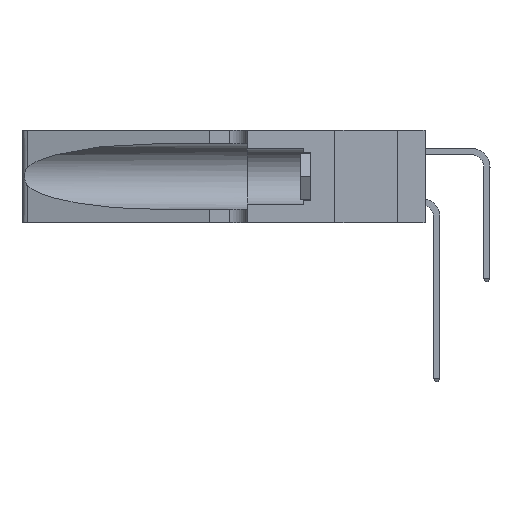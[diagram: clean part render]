
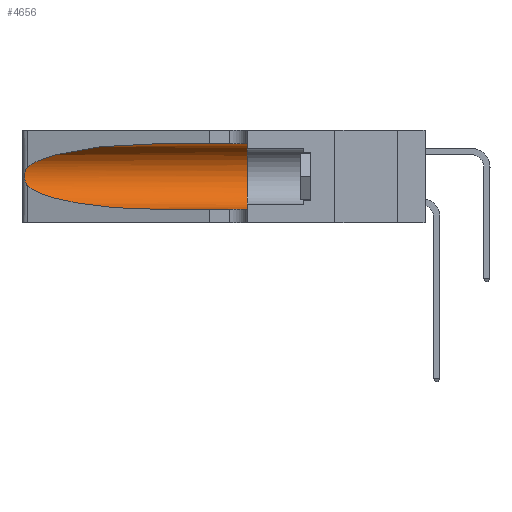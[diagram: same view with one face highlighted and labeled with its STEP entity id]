
A CAD part, left-side view. The second image highlights one B-rep face of the part: STEP entity #4656.
In plain terms, the highlighted cylindrical face has radius 3.308 mm (diameter 6.617 mm), a partial arc.
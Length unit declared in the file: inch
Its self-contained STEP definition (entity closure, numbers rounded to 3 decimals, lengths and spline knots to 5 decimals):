
#971 = EDGE_CURVE ( 'NONE', #30730, #7236, #8012, .T. ) ;
#1687 = VERTEX_POINT ( 'NONE', #6755 ) ;
#1723 = CARTESIAN_POINT ( 'NONE',  ( 0.1305, 1.61858, 0.05475 ) ) ;
#2503 = VECTOR ( 'NONE', #32444, 39.37008 ) ;
#2796 = VERTEX_POINT ( 'NONE', #14211 ) ;
#4023 = CARTESIAN_POINT ( 'NONE',  ( 0.1305, 0.72297, 0.31525 ) ) ;
#4656 = ADVANCED_FACE ( 'NONE', ( #18429 ), #18803, .F. ) ;
#6582 = EDGE_CURVE ( 'NONE', #15740, #2796, #26088, .T. ) ;
#6755 = CARTESIAN_POINT ( 'NONE',  ( 0.1305, 0.35, 0.31525 ) ) ;
#7236 = VERTEX_POINT ( 'NONE', #12376 ) ;
#7680 = CARTESIAN_POINT ( 'NONE',  ( 0.25487, 1.22718, 0.14631 ) ) ;
#8012 =( BOUNDED_CURVE ( )  B_SPLINE_CURVE ( 3, ( #4023, #9472, #24943, #17368 ),
 .UNSPECIFIED., .F., .T. ) 
 B_SPLINE_CURVE_WITH_KNOTS ( ( 4, 4 ),
 ( 1.5708, 2.84003 ),
 .UNSPECIFIED. ) 
 CURVE ( )  GEOMETRIC_REPRESENTATION_ITEM ( )  RATIONAL_B_SPLINE_CURVE ( ( 1., 0.87, 0.87, 1. ) ) 
 REPRESENTATION_ITEM ( '' )  );
#9037 = CIRCLE ( 'NONE', #13797, 0.13025 ) ;
#9049 = DIRECTION ( 'NONE',  ( 0., 0., 1. ) ) ;
#9266 = CARTESIAN_POINT ( 'NONE',  ( 0.1305, 0.72297, 0.31525 ) ) ;
#9472 = CARTESIAN_POINT ( 'NONE',  ( 0.18966, 0.96281, 0.31525 ) ) ;
#10345 = ORIENTED_EDGE ( 'NONE', *, *, #21087, .T. ) ;
#11598 = LINE ( 'NONE', #26749, #31952 ) ;
#11802 = CARTESIAN_POINT ( 'NONE',  ( 0.26075, 1.23896, 0.19203 ) ) ;
#11924 = CARTESIAN_POINT ( 'NONE',  ( 0.25639, 1.23186, 0.15144 ) ) ;
#12041 = CARTESIAN_POINT ( 'NONE',  ( 0.25487, 1.22718, 0.22369 ) ) ;
#12376 = CARTESIAN_POINT ( 'NONE',  ( 0.25487, 1.22718, 0.22369 ) ) ;
#12915 = EDGE_CURVE ( 'NONE', #30730, #1687, #11598, .T. ) ;
#13797 = AXIS2_PLACEMENT_3D ( 'NONE', #30279, #24888, #9049 ) ;
#13866 = CARTESIAN_POINT ( 'NONE',  ( 0.25487, 1.22718, 0.14631 ) ) ;
#13899 = DIRECTION ( 'NONE',  ( 0., -1., 0. ) ) ;
#14119 = CARTESIAN_POINT ( 'NONE',  ( 0.1305, 1.61858, 0.185 ) ) ;
#14211 = CARTESIAN_POINT ( 'NONE',  ( 0.1305, 0.35, 0.05475 ) ) ;
#15256 =( BOUNDED_CURVE ( )  B_SPLINE_CURVE ( 3, ( #7680, #18378, #34017, #26201 ),
 .UNSPECIFIED., .F., .F. ) 
 B_SPLINE_CURVE_WITH_KNOTS ( ( 4, 4 ),
 ( 3.44316, 4.71239 ),
 .UNSPECIFIED. ) 
 CURVE ( )  GEOMETRIC_REPRESENTATION_ITEM ( )  RATIONAL_B_SPLINE_CURVE ( ( 1., 0.87, 0.87, 1. ) ) 
 REPRESENTATION_ITEM ( '' )  );
#15740 = VERTEX_POINT ( 'NONE', #21078 ) ;
#16874 = EDGE_CURVE ( 'NONE', #7236, #31342, #18451, .T. ) ;
#16885 = ORIENTED_EDGE ( 'NONE', *, *, #12915, .F. ) ;
#17141 = CARTESIAN_POINT ( 'NONE',  ( 0.25789, 1.23486, 0.15765 ) ) ;
#17258 = CARTESIAN_POINT ( 'NONE',  ( 0.26017, 1.23833, 0.17102 ) ) ;
#17368 = CARTESIAN_POINT ( 'NONE',  ( 0.25487, 1.22718, 0.22369 ) ) ;
#18378 = CARTESIAN_POINT ( 'NONE',  ( 0.2373, 1.15595, 0.08982 ) ) ;
#18429 = FACE_OUTER_BOUND ( 'NONE', #32497, .T. ) ;
#18451 = B_SPLINE_CURVE_WITH_KNOTS ( 'NONE', 3,
 ( #12041, #24957, #27506, #27621, #22561, #25093, #11802, #30221, #17258, #30351, #17141, #11924, #27741, #30464 ),
 .UNSPECIFIED., .F., .F.,
 ( 4, 2, 2, 2, 2, 2, 4 ),
 ( 0., 0.00027, 0.00053, 0.00107, 0.0016, 0.00187, 0.00214 ),
 .UNSPECIFIED. ) ;
#18803 = CYLINDRICAL_SURFACE ( 'NONE', #33532, 0.13025 ) ;
#20384 = EDGE_CURVE ( 'NONE', #1687, #2796, #9037, .T. ) ;
#21078 = CARTESIAN_POINT ( 'NONE',  ( 0.1305, 0.72297, 0.05475 ) ) ;
#21087 = EDGE_CURVE ( 'NONE', #31342, #15740, #15256, .T. ) ;
#21212 = ORIENTED_EDGE ( 'NONE', *, *, #6582, .T. ) ;
#22356 = DIRECTION ( 'NONE',  ( 0., -1., 0. ) ) ;
#22364 = ORIENTED_EDGE ( 'NONE', *, *, #16874, .T. ) ;
#22561 = CARTESIAN_POINT ( 'NONE',  ( 0.25854, 1.2359, 0.20912 ) ) ;
#24888 = DIRECTION ( 'NONE',  ( 0., 1., 0. ) ) ;
#24943 = CARTESIAN_POINT ( 'NONE',  ( 0.2373, 1.15595, 0.28018 ) ) ;
#24957 = CARTESIAN_POINT ( 'NONE',  ( 0.25555, 1.22994, 0.2215 ) ) ;
#25093 = CARTESIAN_POINT ( 'NONE',  ( 0.26018, 1.23835, 0.19895 ) ) ;
#26088 = LINE ( 'NONE', #1723, #2503 ) ;
#26201 = CARTESIAN_POINT ( 'NONE',  ( 0.1305, 0.72297, 0.05475 ) ) ;
#26749 = CARTESIAN_POINT ( 'NONE',  ( 0.1305, 1.61858, 0.31525 ) ) ;
#27506 = CARTESIAN_POINT ( 'NONE',  ( 0.25639, 1.23184, 0.21858 ) ) ;
#27621 = CARTESIAN_POINT ( 'NONE',  ( 0.25787, 1.23484, 0.2124 ) ) ;
#27741 = CARTESIAN_POINT ( 'NONE',  ( 0.25555, 1.22993, 0.14849 ) ) ;
#28858 = ORIENTED_EDGE ( 'NONE', *, *, #20384, .F. ) ;
#30221 = CARTESIAN_POINT ( 'NONE',  ( 0.26075, 1.23896, 0.178 ) ) ;
#30279 = CARTESIAN_POINT ( 'NONE',  ( 0.1305, 0.35, 0.185 ) ) ;
#30351 = CARTESIAN_POINT ( 'NONE',  ( 0.25856, 1.23593, 0.16098 ) ) ;
#30464 = CARTESIAN_POINT ( 'NONE',  ( 0.25487, 1.22718, 0.14631 ) ) ;
#30502 = ORIENTED_EDGE ( 'NONE', *, *, #971, .T. ) ;
#30730 = VERTEX_POINT ( 'NONE', #9266 ) ;
#31342 = VERTEX_POINT ( 'NONE', #13866 ) ;
#31952 = VECTOR ( 'NONE', #22356, 39.37008 ) ;
#32441 = DIRECTION ( 'NONE',  ( 0., 0., -1. ) ) ;
#32444 = DIRECTION ( 'NONE',  ( 0., -1., 0. ) ) ;
#32497 = EDGE_LOOP ( 'NONE', ( #30502, #22364, #10345, #21212, #28858, #16885 ) ) ;
#33532 = AXIS2_PLACEMENT_3D ( 'NONE', #14119, #13899, #32441 ) ;
#34017 = CARTESIAN_POINT ( 'NONE',  ( 0.18966, 0.96281, 0.05475 ) ) ;
